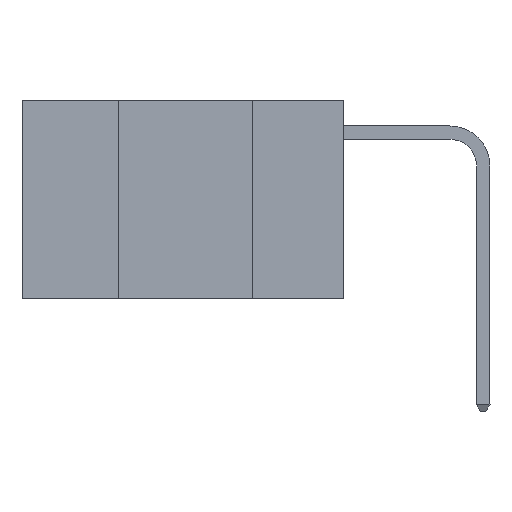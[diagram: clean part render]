
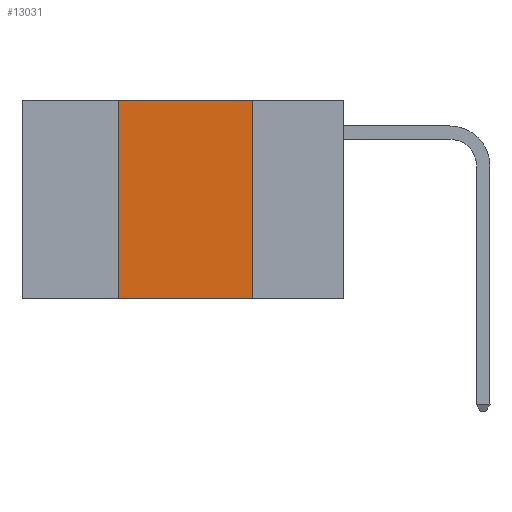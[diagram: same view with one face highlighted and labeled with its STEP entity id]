
A CAD part, left-side view. The second image highlights one B-rep face of the part: STEP entity #13031.
In plain terms, the highlighted planar face has unit normal (-1, 0, 0).
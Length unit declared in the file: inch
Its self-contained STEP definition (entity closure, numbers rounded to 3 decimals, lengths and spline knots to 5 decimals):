
#291 = CARTESIAN_POINT ( 'NONE',  ( 0., 0.17, -0.37 ) ) ;
#959 = VERTEX_POINT ( 'NONE', #291 ) ;
#1614 = EDGE_CURVE ( 'NONE', #4007, #959, #11795, .T. ) ;
#1813 = CARTESIAN_POINT ( 'NONE',  ( 0., 0.42, -0.37 ) ) ;
#1907 = VERTEX_POINT ( 'NONE', #6007 ) ;
#2706 = EDGE_CURVE ( 'NONE', #4007, #1907, #13740, .T. ) ;
#3795 = ORIENTED_EDGE ( 'NONE', *, *, #1614, .T. ) ;
#4007 = VERTEX_POINT ( 'NONE', #1813 ) ;
#4646 = CARTESIAN_POINT ( 'NONE',  ( 0., 0.17, 0. ) ) ;
#5158 = DIRECTION ( 'NONE',  ( 1., 0., 0. ) ) ;
#5719 = DIRECTION ( 'NONE',  ( 0., 0., 1. ) ) ;
#5889 = DIRECTION ( 'NONE',  ( 0., -1., 0. ) ) ;
#6007 = CARTESIAN_POINT ( 'NONE',  ( 0., 0.42, 0. ) ) ;
#6091 = CARTESIAN_POINT ( 'NONE',  ( 0., 0.6, 0. ) ) ;
#6099 = VERTEX_POINT ( 'NONE', #4646 ) ;
#7470 = VECTOR ( 'NONE', #17125, 39.37008 ) ;
#8198 = DIRECTION ( 'NONE',  ( 0., 0., -1. ) ) ;
#8243 = CARTESIAN_POINT ( 'NONE',  ( 0., 0.6, 0. ) ) ;
#8362 = CARTESIAN_POINT ( 'NONE',  ( 0., 0.17, 0. ) ) ;
#8743 = AXIS2_PLACEMENT_3D ( 'NONE', #6091, #5158, #8198 ) ;
#9791 = ORIENTED_EDGE ( 'NONE', *, *, #2706, .F. ) ;
#9840 = DIRECTION ( 'NONE',  ( 0., 0., -1. ) ) ;
#10411 = EDGE_LOOP ( 'NONE', ( #13203, #16949, #9791, #3795 ) ) ;
#10975 = EDGE_CURVE ( 'NONE', #6099, #959, #12297, .T. ) ;
#11531 = VECTOR ( 'NONE', #5719, 39.37008 ) ;
#11794 = PLANE ( 'NONE',  #8743 ) ;
#11795 = LINE ( 'NONE', #16873, #7470 ) ;
#11971 = FACE_OUTER_BOUND ( 'NONE', #10411, .T. ) ;
#12297 = LINE ( 'NONE', #8362, #13704 ) ;
#13031 = ADVANCED_FACE ( 'NONE', ( #11971 ), #11794, .F. ) ;
#13203 = ORIENTED_EDGE ( 'NONE', *, *, #10975, .F. ) ;
#13704 = VECTOR ( 'NONE', #9840, 39.37008 ) ;
#13740 = LINE ( 'NONE', #14962, #11531 ) ;
#14619 = VECTOR ( 'NONE', #5889, 39.37008 ) ;
#14962 = CARTESIAN_POINT ( 'NONE',  ( 0., 0.42, 0. ) ) ;
#15370 = EDGE_CURVE ( 'NONE', #1907, #6099, #16279, .T. ) ;
#16279 = LINE ( 'NONE', #8243, #14619 ) ;
#16873 = CARTESIAN_POINT ( 'NONE',  ( 0., 0.6, -0.37 ) ) ;
#16949 = ORIENTED_EDGE ( 'NONE', *, *, #15370, .F. ) ;
#17125 = DIRECTION ( 'NONE',  ( 0., -1., 0. ) ) ;
